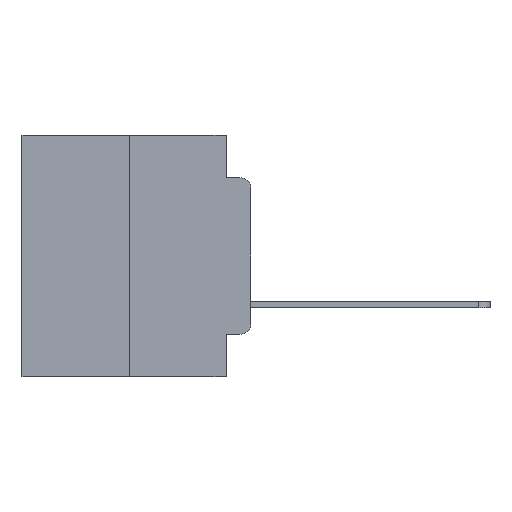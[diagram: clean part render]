
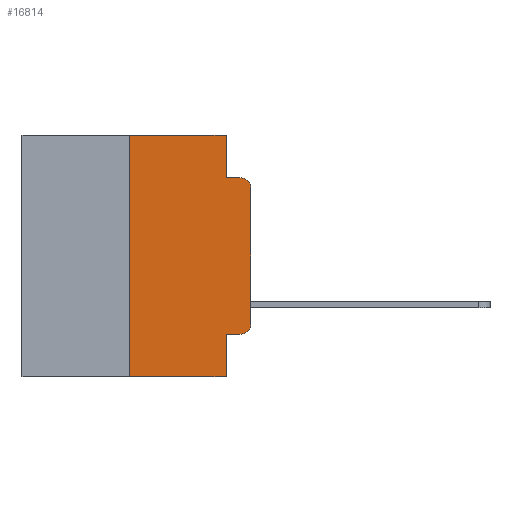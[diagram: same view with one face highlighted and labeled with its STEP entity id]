
A CAD part, left-side view. The second image highlights one B-rep face of the part: STEP entity #16814.
In plain terms, the highlighted planar face has unit normal (-1, 0, 0).
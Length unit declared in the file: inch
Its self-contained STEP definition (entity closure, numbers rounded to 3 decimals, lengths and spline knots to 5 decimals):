
#22 = AXIS2_PLACEMENT_3D ( 'NONE', #22949, #24959, #4803 ) ;
#221 = VERTEX_POINT ( 'NONE', #11428 ) ;
#318 = VERTEX_POINT ( 'NONE', #7640 ) ;
#390 = AXIS2_PLACEMENT_3D ( 'NONE', #13709, #3635, #17660 ) ;
#891 = VECTOR ( 'NONE', #3806, 39.37008 ) ;
#1023 = VECTOR ( 'NONE', #8310, 39.37008 ) ;
#1243 = EDGE_CURVE ( 'NONE', #221, #2123, #4254, .T. ) ;
#1745 = PLANE ( 'NONE',  #24711 ) ;
#1863 = CARTESIAN_POINT ( 'NONE',  ( 0., 0.02, -0.4115 ) ) ;
#1950 = ORIENTED_EDGE ( 'NONE', *, *, #20968, .T. ) ;
#1956 = CARTESIAN_POINT ( 'NONE',  ( 0., 0.051, 0. ) ) ;
#2123 = VERTEX_POINT ( 'NONE', #1863 ) ;
#2165 = DIRECTION ( 'NONE',  ( 0., 0., -1. ) ) ;
#3635 = DIRECTION ( 'NONE',  ( -1., 0., 0. ) ) ;
#3668 = DIRECTION ( 'NONE',  ( 0., 0., 1. ) ) ;
#3806 = DIRECTION ( 'NONE',  ( 0., -1., 0. ) ) ;
#4254 = LINE ( 'NONE', #20579, #5577 ) ;
#4423 = ORIENTED_EDGE ( 'NONE', *, *, #5257, .T. ) ;
#4695 = EDGE_CURVE ( 'NONE', #10501, #25591, #17253, .T. ) ;
#4803 = DIRECTION ( 'NONE',  ( 0., 0., -1. ) ) ;
#5257 = EDGE_CURVE ( 'NONE', #25635, #5469, #14350, .T. ) ;
#5469 = VERTEX_POINT ( 'NONE', #15602 ) ;
#5577 = VECTOR ( 'NONE', #20330, 39.37008 ) ;
#5592 = FACE_OUTER_BOUND ( 'NONE', #22966, .T. ) ;
#5703 = CARTESIAN_POINT ( 'NONE',  ( 0., 0.473, 0. ) ) ;
#7106 = VECTOR ( 'NONE', #2165, 39.37008 ) ;
#7640 = CARTESIAN_POINT ( 'NONE',  ( 0., 0.051, -0.5 ) ) ;
#7809 = DIRECTION ( 'NONE',  ( 0., 0., -1. ) ) ;
#7848 = CARTESIAN_POINT ( 'NONE',  ( 0., 0.473, 0. ) ) ;
#8310 = DIRECTION ( 'NONE',  ( 0., -1., 0. ) ) ;
#8496 = EDGE_CURVE ( 'NONE', #16272, #10501, #16401, .T. ) ;
#8512 = ORIENTED_EDGE ( 'NONE', *, *, #17601, .F. ) ;
#9304 = ORIENTED_EDGE ( 'NONE', *, *, #4695, .F. ) ;
#9886 = DIRECTION ( 'NONE',  ( 0., 0., -1. ) ) ;
#10118 = VERTEX_POINT ( 'NONE', #19407 ) ;
#10501 = VERTEX_POINT ( 'NONE', #11837 ) ;
#11258 = EDGE_CURVE ( 'NONE', #10118, #16272, #17984, .T. ) ;
#11428 = CARTESIAN_POINT ( 'NONE',  ( 0., 0.051, -0.4115 ) ) ;
#11837 = CARTESIAN_POINT ( 'NONE',  ( 0., 0.051, 0. ) ) ;
#13709 = CARTESIAN_POINT ( 'NONE',  ( 0., 0.02, -0.1085 ) ) ;
#13848 = CARTESIAN_POINT ( 'NONE',  ( 0., 0., 0. ) ) ;
#13889 = ORIENTED_EDGE ( 'NONE', *, *, #11258, .F. ) ;
#14152 = VECTOR ( 'NONE', #23695, 39.37008 ) ;
#14350 = CIRCLE ( 'NONE', #390, 0.02 ) ;
#14539 = CARTESIAN_POINT ( 'NONE',  ( 0., 0.051, -0.0885 ) ) ;
#15565 = ORIENTED_EDGE ( 'NONE', *, *, #8496, .F. ) ;
#15602 = CARTESIAN_POINT ( 'NONE',  ( 0., 0.02, -0.0885 ) ) ;
#16272 = VERTEX_POINT ( 'NONE', #19722 ) ;
#16401 = LINE ( 'NONE', #5703, #23751 ) ;
#16503 = ORIENTED_EDGE ( 'NONE', *, *, #21891, .T. ) ;
#16814 = ADVANCED_FACE ( 'NONE', ( #5592 ), #1745, .F. ) ;
#17253 = LINE ( 'NONE', #1956, #21779 ) ;
#17601 = EDGE_CURVE ( 'NONE', #25591, #5469, #17977, .T. ) ;
#17660 = DIRECTION ( 'NONE',  ( 0., 0., -1. ) ) ;
#17969 = CIRCLE ( 'NONE', #22, 0.02 ) ;
#17977 = LINE ( 'NONE', #14539, #1023 ) ;
#17984 = LINE ( 'NONE', #21584, #14152 ) ;
#18761 = CARTESIAN_POINT ( 'NONE',  ( 0., 0.051, -0.0885 ) ) ;
#19115 = ORIENTED_EDGE ( 'NONE', *, *, #24679, .T. ) ;
#19349 = ORIENTED_EDGE ( 'NONE', *, *, #1243, .T. ) ;
#19407 = CARTESIAN_POINT ( 'NONE',  ( 0., 0.25, -0.5 ) ) ;
#19714 = LINE ( 'NONE', #13848, #21652 ) ;
#19722 = CARTESIAN_POINT ( 'NONE',  ( 0., 0.25, 0. ) ) ;
#20317 = CARTESIAN_POINT ( 'NONE',  ( 0., 0.051, 0. ) ) ;
#20330 = DIRECTION ( 'NONE',  ( 0., -1., 0. ) ) ;
#20413 = LINE ( 'NONE', #24224, #891 ) ;
#20520 = LINE ( 'NONE', #20317, #7106 ) ;
#20579 = CARTESIAN_POINT ( 'NONE',  ( 0., 0.051, -0.4115 ) ) ;
#20968 = EDGE_CURVE ( 'NONE', #10118, #318, #20413, .T. ) ;
#21094 = EDGE_CURVE ( 'NONE', #221, #318, #20520, .T. ) ;
#21167 = CARTESIAN_POINT ( 'NONE',  ( 0., 0., -0.3915 ) ) ;
#21584 = CARTESIAN_POINT ( 'NONE',  ( 0., 0.25, 0. ) ) ;
#21652 = VECTOR ( 'NONE', #3668, 39.37008 ) ;
#21779 = VECTOR ( 'NONE', #7809, 39.37008 ) ;
#21891 = EDGE_CURVE ( 'NONE', #2123, #26190, #17969, .T. ) ;
#22938 = ORIENTED_EDGE ( 'NONE', *, *, #21094, .F. ) ;
#22949 = CARTESIAN_POINT ( 'NONE',  ( 0., 0.02, -0.3915 ) ) ;
#22966 = EDGE_LOOP ( 'NONE', ( #19115, #4423, #8512, #9304, #15565, #13889, #1950, #22938, #19349, #16503 ) ) ;
#23154 = CARTESIAN_POINT ( 'NONE',  ( 0., 0., -0.1085 ) ) ;
#23695 = DIRECTION ( 'NONE',  ( 0., 0., 1. ) ) ;
#23751 = VECTOR ( 'NONE', #25949, 39.37008 ) ;
#24224 = CARTESIAN_POINT ( 'NONE',  ( 0., 0.473, -0.5 ) ) ;
#24679 = EDGE_CURVE ( 'NONE', #26190, #25635, #19714, .T. ) ;
#24711 = AXIS2_PLACEMENT_3D ( 'NONE', #7848, #26293, #9886 ) ;
#24959 = DIRECTION ( 'NONE',  ( -1., 0., 0. ) ) ;
#25591 = VERTEX_POINT ( 'NONE', #18761 ) ;
#25635 = VERTEX_POINT ( 'NONE', #23154 ) ;
#25949 = DIRECTION ( 'NONE',  ( 0., -1., 0. ) ) ;
#26190 = VERTEX_POINT ( 'NONE', #21167 ) ;
#26293 = DIRECTION ( 'NONE',  ( 1., 0., 0. ) ) ;
